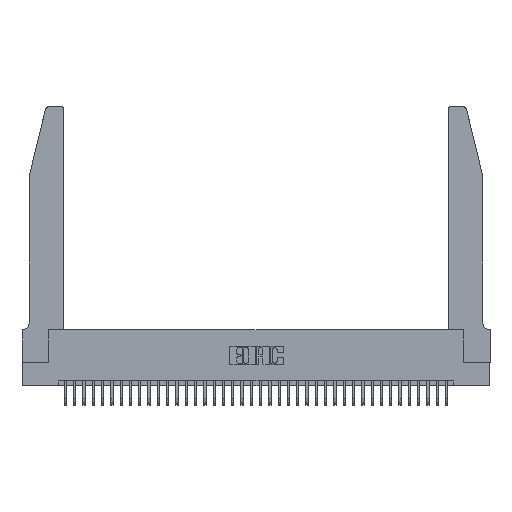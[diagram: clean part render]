
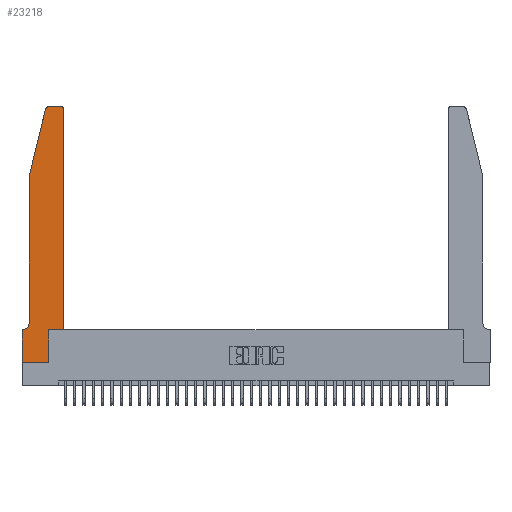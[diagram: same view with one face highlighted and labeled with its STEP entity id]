
A CAD part, top view. The second image highlights one B-rep face of the part: STEP entity #23218.
In plain terms, the highlighted planar face has unit normal (0, 0, 1).
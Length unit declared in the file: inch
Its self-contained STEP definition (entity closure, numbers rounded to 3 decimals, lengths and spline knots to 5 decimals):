
#1360 = VERTEX_POINT ( 'NONE', #7609 ) ;
#1938 = ORIENTED_EDGE ( 'NONE', *, *, #4758, .T. ) ;
#2642 = CARTESIAN_POINT ( 'NONE',  ( 0.284, 2.72, 0.37 ) ) ;
#2725 = CARTESIAN_POINT ( 'NONE',  ( 0.0755, 0.35, 0.37 ) ) ;
#2901 = CARTESIAN_POINT ( 'NONE',  ( 0.0755, 2., 0.37 ) ) ;
#2910 = DIRECTION ( 'NONE',  ( 1., 0., 0. ) ) ;
#2912 = DIRECTION ( 'NONE',  ( 0., 1., 0. ) ) ;
#3087 = LINE ( 'NONE', #2901, #18393 ) ;
#3163 = VERTEX_POINT ( 'NONE', #13384 ) ;
#3380 = CARTESIAN_POINT ( 'NONE',  ( 0.0755, 2., 0.37 ) ) ;
#4262 = CIRCLE ( 'NONE', #38917, 0.07 ) ;
#4571 = CARTESIAN_POINT ( 'NONE',  ( 0., 0., 0.37 ) ) ;
#4758 = EDGE_CURVE ( 'NONE', #32246, #20527, #14200, .T. ) ;
#5290 = DIRECTION ( 'NONE',  ( -1., 0., 0. ) ) ;
#5715 = DIRECTION ( 'NONE',  ( 1., 0., 0. ) ) ;
#5956 = LINE ( 'NONE', #4571, #37332 ) ;
#5984 = DIRECTION ( 'NONE',  ( 0., -1., 0. ) ) ;
#6055 = VECTOR ( 'NONE', #18611, 39.37008 ) ;
#6181 = VERTEX_POINT ( 'NONE', #19039 ) ;
#6388 = CARTESIAN_POINT ( 'NONE',  ( 0.4505, 0.35, 0.37 ) ) ;
#6666 = EDGE_CURVE ( 'NONE', #3163, #18743, #21674, .T. ) ;
#7386 = DIRECTION ( 'NONE',  ( 1., 0., 0. ) ) ;
#7550 = VECTOR ( 'NONE', #33742, 39.37008 ) ;
#7609 = CARTESIAN_POINT ( 'NONE',  ( 0.2865, 0.35, 0.37 ) ) ;
#7633 = DIRECTION ( 'NONE',  ( 0., -1., 0. ) ) ;
#7862 = ORIENTED_EDGE ( 'NONE', *, *, #36693, .T. ) ;
#8416 = ORIENTED_EDGE ( 'NONE', *, *, #25860, .T. ) ;
#8557 = DIRECTION ( 'NONE',  ( 0., 0., -1. ) ) ;
#8643 = ORIENTED_EDGE ( 'NONE', *, *, #21138, .T. ) ;
#8807 = CARTESIAN_POINT ( 'NONE',  ( 0.4505, 0.35, 0.37 ) ) ;
#9375 = EDGE_CURVE ( 'NONE', #20771, #18310, #4262, .T. ) ;
#9942 = CARTESIAN_POINT ( 'NONE',  ( 0.4205, 2.72, 0.37 ) ) ;
#10687 = EDGE_CURVE ( 'NONE', #6181, #22627, #31820, .T. ) ;
#11390 = VECTOR ( 'NONE', #13791, 39.37008 ) ;
#11713 = VERTEX_POINT ( 'NONE', #14673 ) ;
#11993 = LINE ( 'NONE', #17435, #26291 ) ;
#12659 = LINE ( 'NONE', #39289, #27885 ) ;
#12967 = VECTOR ( 'NONE', #2910, 39.37008 ) ;
#13003 = DIRECTION ( 'NONE',  ( 1., 0., 0. ) ) ;
#13074 = ORIENTED_EDGE ( 'NONE', *, *, #38520, .T. ) ;
#13220 = AXIS2_PLACEMENT_3D ( 'NONE', #2642, #24026, #5715 ) ;
#13271 = ORIENTED_EDGE ( 'NONE', *, *, #25308, .T. ) ;
#13384 = CARTESIAN_POINT ( 'NONE',  ( 0.4505, 2.72, 0.37 ) ) ;
#13791 = DIRECTION ( 'NONE',  ( 0., 1., 0. ) ) ;
#14200 = LINE ( 'NONE', #3380, #6055 ) ;
#14673 = CARTESIAN_POINT ( 'NONE',  ( 0.284, 2.75, 0.37 ) ) ;
#15951 = VECTOR ( 'NONE', #27151, 39.37008 ) ;
#16606 = ORIENTED_EDGE ( 'NONE', *, *, #6666, .T. ) ;
#17435 = CARTESIAN_POINT ( 'NONE',  ( 0.2605, 2.75, 0.37 ) ) ;
#18021 = EDGE_LOOP ( 'NONE', ( #8643, #13074, #1938, #13271, #25068, #8416, #22702, #35268, #32940, #7862, #37479, #16606 ) ) ;
#18022 = CARTESIAN_POINT ( 'NONE',  ( 0.4205, 2.75, 0.37 ) ) ;
#18310 = VERTEX_POINT ( 'NONE', #35888 ) ;
#18393 = VECTOR ( 'NONE', #5984, 39.37008 ) ;
#18611 = DIRECTION ( 'NONE',  ( -0.239, -0.971, 0. ) ) ;
#18743 = VERTEX_POINT ( 'NONE', #18022 ) ;
#18750 = AXIS2_PLACEMENT_3D ( 'NONE', #22635, #25685, #7386 ) ;
#19039 = CARTESIAN_POINT ( 'NONE',  ( 0., 0., 0.37 ) ) ;
#19549 = PLANE ( 'NONE',  #18750 ) ;
#19977 = CIRCLE ( 'NONE', #13220, 0.03 ) ;
#19989 = CARTESIAN_POINT ( 'NONE',  ( 0.2865, 0., 0.37 ) ) ;
#20527 = VERTEX_POINT ( 'NONE', #29182 ) ;
#20771 = VERTEX_POINT ( 'NONE', #30604 ) ;
#21138 = EDGE_CURVE ( 'NONE', #18743, #11713, #11993, .T. ) ;
#21674 = CIRCLE ( 'NONE', #21975, 0.03 ) ;
#21975 = AXIS2_PLACEMENT_3D ( 'NONE', #9942, #31204, #13003 ) ;
#22627 = VERTEX_POINT ( 'NONE', #19989 ) ;
#22635 = CARTESIAN_POINT ( 'NONE',  ( 0., 0.35, 0.37 ) ) ;
#22702 = ORIENTED_EDGE ( 'NONE', *, *, #33617, .T. ) ;
#23218 = ADVANCED_FACE ( 'NONE', ( #28075 ), #19549, .T. ) ;
#24026 = DIRECTION ( 'NONE',  ( 0., 0., 1. ) ) ;
#25068 = ORIENTED_EDGE ( 'NONE', *, *, #9375, .T. ) ;
#25308 = EDGE_CURVE ( 'NONE', #20527, #20771, #3087, .T. ) ;
#25378 = VERTEX_POINT ( 'NONE', #6388 ) ;
#25685 = DIRECTION ( 'NONE',  ( 0., 0., 1. ) ) ;
#25860 = EDGE_CURVE ( 'NONE', #18310, #34968, #32088, .T. ) ;
#26291 = VECTOR ( 'NONE', #5290, 39.37008 ) ;
#26826 = CARTESIAN_POINT ( 'NONE',  ( 0.0055, 0.42, 0.37 ) ) ;
#27151 = DIRECTION ( 'NONE',  ( -1., 0., 0. ) ) ;
#27885 = VECTOR ( 'NONE', #2912, 39.37008 ) ;
#28075 = FACE_OUTER_BOUND ( 'NONE', #18021, .T. ) ;
#29138 = LINE ( 'NONE', #8807, #12967 ) ;
#29182 = CARTESIAN_POINT ( 'NONE',  ( 0.0755, 2., 0.37 ) ) ;
#29503 = CARTESIAN_POINT ( 'NONE',  ( 0., 0.35, 0.37 ) ) ;
#29857 = DIRECTION ( 'NONE',  ( -1., 0., 0. ) ) ;
#30604 = CARTESIAN_POINT ( 'NONE',  ( 0.0755, 0.42, 0.37 ) ) ;
#31204 = DIRECTION ( 'NONE',  ( 0., 0., 1. ) ) ;
#31820 = LINE ( 'NONE', #36770, #7550 ) ;
#31965 = CARTESIAN_POINT ( 'NONE',  ( 0.2865, 0.35, 0.37 ) ) ;
#32088 = LINE ( 'NONE', #2725, #15951 ) ;
#32246 = VERTEX_POINT ( 'NONE', #34755 ) ;
#32940 = ORIENTED_EDGE ( 'NONE', *, *, #38281, .T. ) ;
#33617 = EDGE_CURVE ( 'NONE', #34968, #6181, #5956, .T. ) ;
#33742 = DIRECTION ( 'NONE',  ( 1., 0., 0. ) ) ;
#33922 = EDGE_CURVE ( 'NONE', #25378, #3163, #12659, .T. ) ;
#34755 = CARTESIAN_POINT ( 'NONE',  ( 0.25487, 2.72718, 0.37 ) ) ;
#34968 = VERTEX_POINT ( 'NONE', #29503 ) ;
#35268 = ORIENTED_EDGE ( 'NONE', *, *, #10687, .T. ) ;
#35622 = LINE ( 'NONE', #31965, #11390 ) ;
#35888 = CARTESIAN_POINT ( 'NONE',  ( 0.0055, 0.35, 0.37 ) ) ;
#36693 = EDGE_CURVE ( 'NONE', #1360, #25378, #29138, .T. ) ;
#36770 = CARTESIAN_POINT ( 'NONE',  ( 0., 0., 0.37 ) ) ;
#37332 = VECTOR ( 'NONE', #7633, 39.37008 ) ;
#37479 = ORIENTED_EDGE ( 'NONE', *, *, #33922, .T. ) ;
#38281 = EDGE_CURVE ( 'NONE', #22627, #1360, #35622, .T. ) ;
#38520 = EDGE_CURVE ( 'NONE', #11713, #32246, #19977, .T. ) ;
#38917 = AXIS2_PLACEMENT_3D ( 'NONE', #26826, #8557, #29857 ) ;
#39289 = CARTESIAN_POINT ( 'NONE',  ( 0.4505, 0.35, 0.37 ) ) ;
